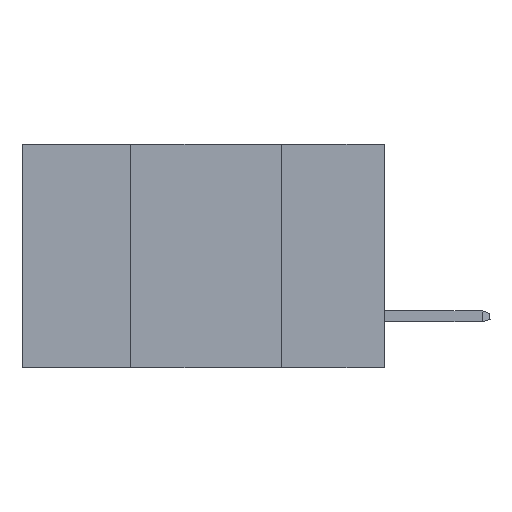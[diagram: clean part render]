
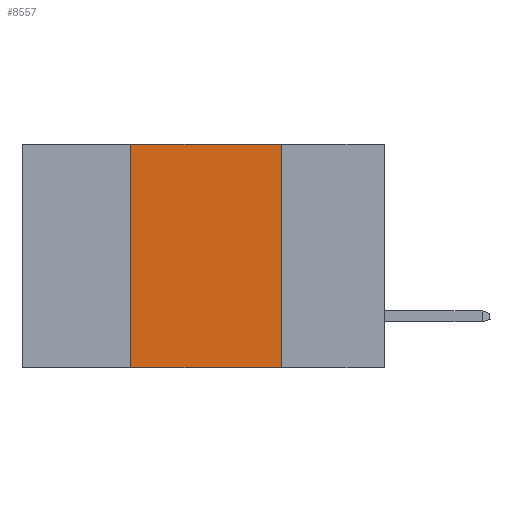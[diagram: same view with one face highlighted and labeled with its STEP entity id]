
A CAD part, left-side view. The second image highlights one B-rep face of the part: STEP entity #8557.
In plain terms, the highlighted planar face has unit normal (-1, 0, 0).
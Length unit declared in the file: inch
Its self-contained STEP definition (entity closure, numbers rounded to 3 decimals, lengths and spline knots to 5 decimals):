
#69 = VECTOR ( 'NONE', #1976, 39.37008 ) ;
#380 = ORIENTED_EDGE ( 'NONE', *, *, #8537, .F. ) ;
#460 = LINE ( 'NONE', #9289, #8790 ) ;
#1083 = CARTESIAN_POINT ( 'NONE',  ( 0., 0.6, -0.37 ) ) ;
#1109 = EDGE_CURVE ( 'NONE', #5721, #5617, #9636, .T. ) ;
#1329 = EDGE_CURVE ( 'NONE', #5721, #2427, #9625, .T. ) ;
#1377 = ORIENTED_EDGE ( 'NONE', *, *, #1109, .F. ) ;
#1815 = DIRECTION ( 'NONE',  ( 0., -1., 0. ) ) ;
#1976 = DIRECTION ( 'NONE',  ( 0., -1., 0. ) ) ;
#2427 = VERTEX_POINT ( 'NONE', #3197 ) ;
#3134 = CARTESIAN_POINT ( 'NONE',  ( 0., 0.17, 0. ) ) ;
#3197 = CARTESIAN_POINT ( 'NONE',  ( 0., 0.17, -0.37 ) ) ;
#3313 = CARTESIAN_POINT ( 'NONE',  ( 0., 0.42, 0. ) ) ;
#3600 = VECTOR ( 'NONE', #11841, 39.37008 ) ;
#4461 = ORIENTED_EDGE ( 'NONE', *, *, #8681, .F. ) ;
#4571 = VECTOR ( 'NONE', #1815, 39.37008 ) ;
#5411 = DIRECTION ( 'NONE',  ( 0., 0., -1. ) ) ;
#5617 = VERTEX_POINT ( 'NONE', #7363 ) ;
#5721 = VERTEX_POINT ( 'NONE', #6206 ) ;
#6206 = CARTESIAN_POINT ( 'NONE',  ( 0., 0.42, -0.37 ) ) ;
#7363 = CARTESIAN_POINT ( 'NONE',  ( 0., 0.42, 0. ) ) ;
#7916 = AXIS2_PLACEMENT_3D ( 'NONE', #10520, #15440, #5411 ) ;
#7987 = LINE ( 'NONE', #14294, #69 ) ;
#8497 = VERTEX_POINT ( 'NONE', #3134 ) ;
#8537 = EDGE_CURVE ( 'NONE', #8497, #2427, #460, .T. ) ;
#8557 = ADVANCED_FACE ( 'NONE', ( #14172 ), #14240, .F. ) ;
#8681 = EDGE_CURVE ( 'NONE', #5617, #8497, #7987, .T. ) ;
#8790 = VECTOR ( 'NONE', #14177, 39.37008 ) ;
#9289 = CARTESIAN_POINT ( 'NONE',  ( 0., 0.17, 0. ) ) ;
#9625 = LINE ( 'NONE', #1083, #4571 ) ;
#9636 = LINE ( 'NONE', #3313, #3600 ) ;
#10520 = CARTESIAN_POINT ( 'NONE',  ( 0., 0.6, 0. ) ) ;
#11841 = DIRECTION ( 'NONE',  ( 0., 0., 1. ) ) ;
#12015 = ORIENTED_EDGE ( 'NONE', *, *, #1329, .T. ) ;
#14172 = FACE_OUTER_BOUND ( 'NONE', #15936, .T. ) ;
#14177 = DIRECTION ( 'NONE',  ( 0., 0., -1. ) ) ;
#14240 = PLANE ( 'NONE',  #7916 ) ;
#14294 = CARTESIAN_POINT ( 'NONE',  ( 0., 0.6, 0. ) ) ;
#15440 = DIRECTION ( 'NONE',  ( 1., 0., 0. ) ) ;
#15936 = EDGE_LOOP ( 'NONE', ( #380, #4461, #1377, #12015 ) ) ;
